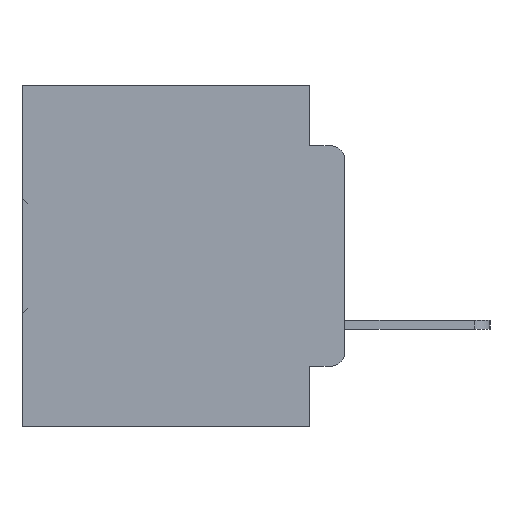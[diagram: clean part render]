
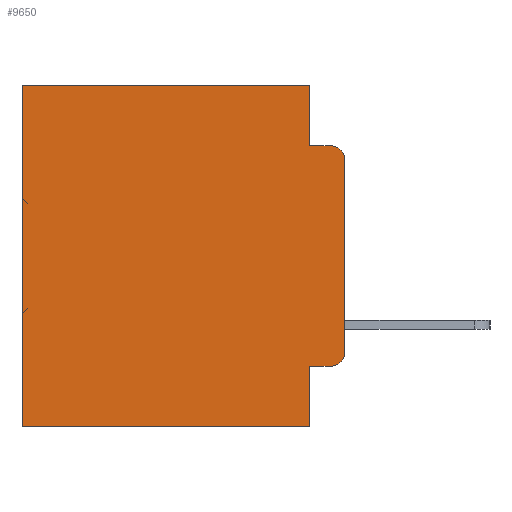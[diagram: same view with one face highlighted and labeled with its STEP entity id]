
A CAD part, left-side view. The second image highlights one B-rep face of the part: STEP entity #9650.
In plain terms, the highlighted planar face has unit normal (-1, 0, 0).
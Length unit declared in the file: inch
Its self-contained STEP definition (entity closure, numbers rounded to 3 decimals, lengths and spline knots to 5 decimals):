
#74 = VECTOR ( 'NONE', #7653, 39.37008 ) ;
#1554 = CARTESIAN_POINT ( 'NONE',  ( 0.298, 0.02, -0.3915 ) ) ;
#1598 = CARTESIAN_POINT ( 'NONE',  ( 0.298, 0.051, 0. ) ) ;
#1653 = DIRECTION ( 'NONE',  ( 0., 0., -1. ) ) ;
#2151 = VECTOR ( 'NONE', #9937, 39.37008 ) ;
#2764 = VECTOR ( 'NONE', #20458, 39.37008 ) ;
#3146 = LINE ( 'NONE', #9214, #2151 ) ;
#3373 = EDGE_CURVE ( 'NONE', #9011, #18430, #17715, .T. ) ;
#3766 = DIRECTION ( 'NONE',  ( -1., 0., 0. ) ) ;
#3833 = EDGE_CURVE ( 'NONE', #7712, #14344, #20337, .T. ) ;
#3955 = EDGE_CURVE ( 'NONE', #12838, #21380, #29982, .T. ) ;
#4903 = EDGE_CURVE ( 'NONE', #21515, #29401, #3146, .T. ) ;
#4989 = DIRECTION ( 'NONE',  ( 0., 0., -1. ) ) ;
#7653 = DIRECTION ( 'NONE',  ( 0., 1., 0. ) ) ;
#7712 = VERTEX_POINT ( 'NONE', #9064 ) ;
#7767 = CARTESIAN_POINT ( 'NONE',  ( 0.298, 0., -0.3915 ) ) ;
#8899 = CARTESIAN_POINT ( 'NONE',  ( 0.298, 0.051, -0.4115 ) ) ;
#9011 = VERTEX_POINT ( 'NONE', #27464 ) ;
#9064 = CARTESIAN_POINT ( 'NONE',  ( 0.298, 0.051, -0.4115 ) ) ;
#9214 = CARTESIAN_POINT ( 'NONE',  ( 0.298, 0., 0. ) ) ;
#9650 = ADVANCED_FACE ( 'NONE', ( #33884 ), #33206, .F. ) ;
#9937 = DIRECTION ( 'NONE',  ( 0., 1., 0. ) ) ;
#10356 = VECTOR ( 'NONE', #25712, 39.37008 ) ;
#10816 = CARTESIAN_POINT ( 'NONE',  ( 0.298, 0., 0. ) ) ;
#11008 = DIRECTION ( 'NONE',  ( 0., 0., -1. ) ) ;
#11797 = EDGE_CURVE ( 'NONE', #27889, #21380, #14094, .T. ) ;
#11930 = LINE ( 'NONE', #36046, #19534 ) ;
#12838 = VERTEX_POINT ( 'NONE', #15752 ) ;
#13979 = DIRECTION ( 'NONE',  ( -1., 0., 0. ) ) ;
#14094 = LINE ( 'NONE', #35918, #34558 ) ;
#14178 = CARTESIAN_POINT ( 'NONE',  ( 0.298, 0.051, 0. ) ) ;
#14344 = VERTEX_POINT ( 'NONE', #36830 ) ;
#14738 = EDGE_CURVE ( 'NONE', #27889, #18430, #31895, .T. ) ;
#15752 = CARTESIAN_POINT ( 'NONE',  ( 0.298, 0.02, -0.4115 ) ) ;
#16642 = DIRECTION ( 'NONE',  ( 1., 0., 0. ) ) ;
#16825 = VECTOR ( 'NONE', #18268, 39.37008 ) ;
#17332 = EDGE_CURVE ( 'NONE', #7712, #12838, #26139, .T. ) ;
#17715 = LINE ( 'NONE', #18379, #16825 ) ;
#18067 = LINE ( 'NONE', #14178, #10356 ) ;
#18268 = DIRECTION ( 'NONE',  ( 0., -1., 0. ) ) ;
#18379 = CARTESIAN_POINT ( 'NONE',  ( 0.298, 0.051, -0.0885 ) ) ;
#18430 = VERTEX_POINT ( 'NONE', #21241 ) ;
#19534 = VECTOR ( 'NONE', #4989, 39.37008 ) ;
#19960 = AXIS2_PLACEMENT_3D ( 'NONE', #1554, #13979, #30084 ) ;
#20337 = LINE ( 'NONE', #1598, #27016 ) ;
#20458 = DIRECTION ( 'NONE',  ( 0., -1., 0. ) ) ;
#21241 = CARTESIAN_POINT ( 'NONE',  ( 0.298, 0.02, -0.0885 ) ) ;
#21380 = VERTEX_POINT ( 'NONE', #7767 ) ;
#21386 = CARTESIAN_POINT ( 'NONE',  ( 0.298, 0.02, -0.1085 ) ) ;
#21515 = VERTEX_POINT ( 'NONE', #31188 ) ;
#22175 = CARTESIAN_POINT ( 'NONE',  ( 0.298, 0., -0.5 ) ) ;
#24275 = DIRECTION ( 'NONE',  ( 0., 0., -1. ) ) ;
#24501 = CARTESIAN_POINT ( 'NONE',  ( 0.298, 0., -0.1085 ) ) ;
#25712 = DIRECTION ( 'NONE',  ( 0., 0., -1. ) ) ;
#26139 = LINE ( 'NONE', #8899, #2764 ) ;
#27004 = ORIENTED_EDGE ( 'NONE', *, *, #11797, .F. ) ;
#27016 = VECTOR ( 'NONE', #1653, 39.37008 ) ;
#27238 = ORIENTED_EDGE ( 'NONE', *, *, #14738, .T. ) ;
#27384 = ORIENTED_EDGE ( 'NONE', *, *, #3373, .F. ) ;
#27464 = CARTESIAN_POINT ( 'NONE',  ( 0.298, 0.051, -0.0885 ) ) ;
#27513 = EDGE_CURVE ( 'NONE', #14344, #36478, #31139, .T. ) ;
#27696 = ORIENTED_EDGE ( 'NONE', *, *, #32732, .F. ) ;
#27889 = VERTEX_POINT ( 'NONE', #24501 ) ;
#28021 = ORIENTED_EDGE ( 'NONE', *, *, #4903, .T. ) ;
#29323 = ORIENTED_EDGE ( 'NONE', *, *, #30733, .T. ) ;
#29401 = VERTEX_POINT ( 'NONE', #33477 ) ;
#29971 = ORIENTED_EDGE ( 'NONE', *, *, #27513, .F. ) ;
#29982 = CIRCLE ( 'NONE', #19960, 0.02 ) ;
#30084 = DIRECTION ( 'NONE',  ( 0., 0., -1. ) ) ;
#30733 = EDGE_CURVE ( 'NONE', #29401, #36478, #11930, .T. ) ;
#31139 = LINE ( 'NONE', #22175, #74 ) ;
#31188 = CARTESIAN_POINT ( 'NONE',  ( 0.298, 0.051, 0. ) ) ;
#31895 = CIRCLE ( 'NONE', #32386, 0.02 ) ;
#32386 = AXIS2_PLACEMENT_3D ( 'NONE', #21386, #3766, #24275 ) ;
#32732 = EDGE_CURVE ( 'NONE', #21515, #9011, #18067, .T. ) ;
#33206 = PLANE ( 'NONE',  #34910 ) ;
#33477 = CARTESIAN_POINT ( 'NONE',  ( 0.298, 0.473, 0. ) ) ;
#33884 = FACE_OUTER_BOUND ( 'NONE', #36138, .T. ) ;
#34215 = ORIENTED_EDGE ( 'NONE', *, *, #3833, .F. ) ;
#34267 = ORIENTED_EDGE ( 'NONE', *, *, #17332, .T. ) ;
#34346 = CARTESIAN_POINT ( 'NONE',  ( 0.298, 0.473, -0.5 ) ) ;
#34558 = VECTOR ( 'NONE', #11008, 39.37008 ) ;
#34910 = AXIS2_PLACEMENT_3D ( 'NONE', #10816, #16642, #35868 ) ;
#35807 = ORIENTED_EDGE ( 'NONE', *, *, #3955, .T. ) ;
#35868 = DIRECTION ( 'NONE',  ( 0., 0., -1. ) ) ;
#35918 = CARTESIAN_POINT ( 'NONE',  ( 0.298, 0., 0. ) ) ;
#36046 = CARTESIAN_POINT ( 'NONE',  ( 0.298, 0.473, 0. ) ) ;
#36138 = EDGE_LOOP ( 'NONE', ( #27004, #27238, #27384, #27696, #28021, #29323, #29971, #34215, #34267, #35807 ) ) ;
#36478 = VERTEX_POINT ( 'NONE', #34346 ) ;
#36830 = CARTESIAN_POINT ( 'NONE',  ( 0.298, 0.051, -0.5 ) ) ;
